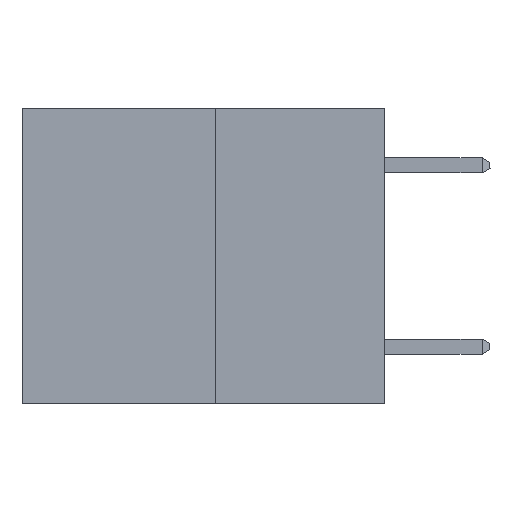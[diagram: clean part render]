
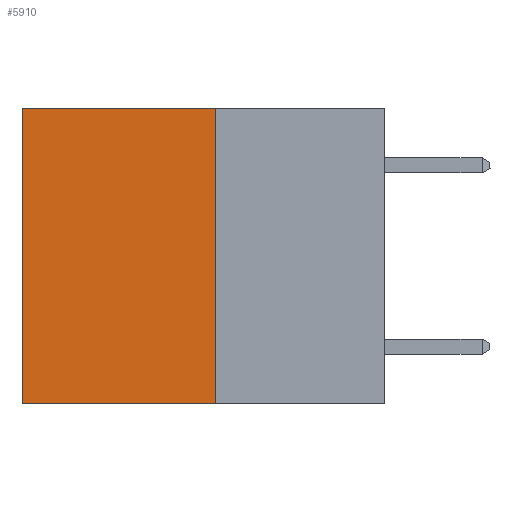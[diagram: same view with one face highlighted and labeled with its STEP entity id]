
A CAD part, left-side view. The second image highlights one B-rep face of the part: STEP entity #5910.
In plain terms, the highlighted planar face has unit normal (-1, 0, 0).
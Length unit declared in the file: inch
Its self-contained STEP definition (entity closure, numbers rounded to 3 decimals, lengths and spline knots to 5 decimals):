
#3016 = LINE ( 'NONE', #24510, #12215 ) ;
#3945 = FACE_OUTER_BOUND ( 'NONE', #21523, .T. ) ;
#5290 = VERTEX_POINT ( 'NONE', #18971 ) ;
#5481 = VERTEX_POINT ( 'NONE', #16877 ) ;
#5910 = ADVANCED_FACE ( 'NONE', ( #3945 ), #23377, .F. ) ;
#6130 = ORIENTED_EDGE ( 'NONE', *, *, #6738, .T. ) ;
#6738 = EDGE_CURVE ( 'NONE', #9419, #5290, #22430, .T. ) ;
#7439 = AXIS2_PLACEMENT_3D ( 'NONE', #19594, #19439, #11404 ) ;
#7853 = EDGE_CURVE ( 'NONE', #9419, #15047, #3016, .T. ) ;
#8755 = DIRECTION ( 'NONE',  ( 0., 1., 0. ) ) ;
#9139 = CARTESIAN_POINT ( 'NONE',  ( 0.3165, 0.6, -0.49 ) ) ;
#9146 = LINE ( 'NONE', #23154, #21821 ) ;
#9419 = VERTEX_POINT ( 'NONE', #20838 ) ;
#9682 = VECTOR ( 'NONE', #23343, 39.37008 ) ;
#9731 = VECTOR ( 'NONE', #8755, 39.37008 ) ;
#10202 = EDGE_CURVE ( 'NONE', #5290, #5481, #14299, .T. ) ;
#11071 = DIRECTION ( 'NONE',  ( 0., 0., -1. ) ) ;
#11404 = DIRECTION ( 'NONE',  ( 0., 0., -1. ) ) ;
#12215 = VECTOR ( 'NONE', #11071, 39.37008 ) ;
#14299 = LINE ( 'NONE', #9139, #9682 ) ;
#15047 = VERTEX_POINT ( 'NONE', #25350 ) ;
#15065 = DIRECTION ( 'NONE',  ( 0., 1., 0. ) ) ;
#16582 = CARTESIAN_POINT ( 'NONE',  ( 0.3165, 0.28, 0. ) ) ;
#16877 = CARTESIAN_POINT ( 'NONE',  ( 0.3165, 0.6, -0.49 ) ) ;
#18971 = CARTESIAN_POINT ( 'NONE',  ( 0.3165, 0.6, 0. ) ) ;
#19439 = DIRECTION ( 'NONE',  ( 1., 0., 0. ) ) ;
#19594 = CARTESIAN_POINT ( 'NONE',  ( 0.3165, 0.28, -0.49 ) ) ;
#19609 = EDGE_CURVE ( 'NONE', #15047, #5481, #9146, .T. ) ;
#20424 = ORIENTED_EDGE ( 'NONE', *, *, #10202, .T. ) ;
#20838 = CARTESIAN_POINT ( 'NONE',  ( 0.3165, 0.28, 0. ) ) ;
#21523 = EDGE_LOOP ( 'NONE', ( #20424, #22989, #24595, #6130 ) ) ;
#21821 = VECTOR ( 'NONE', #15065, 39.37008 ) ;
#22430 = LINE ( 'NONE', #16582, #9731 ) ;
#22989 = ORIENTED_EDGE ( 'NONE', *, *, #19609, .F. ) ;
#23154 = CARTESIAN_POINT ( 'NONE',  ( 0.3165, 0.28, -0.49 ) ) ;
#23343 = DIRECTION ( 'NONE',  ( 0., 0., -1. ) ) ;
#23377 = PLANE ( 'NONE',  #7439 ) ;
#24510 = CARTESIAN_POINT ( 'NONE',  ( 0.3165, 0.28, -0.49 ) ) ;
#24595 = ORIENTED_EDGE ( 'NONE', *, *, #7853, .F. ) ;
#25350 = CARTESIAN_POINT ( 'NONE',  ( 0.3165, 0.28, -0.49 ) ) ;
